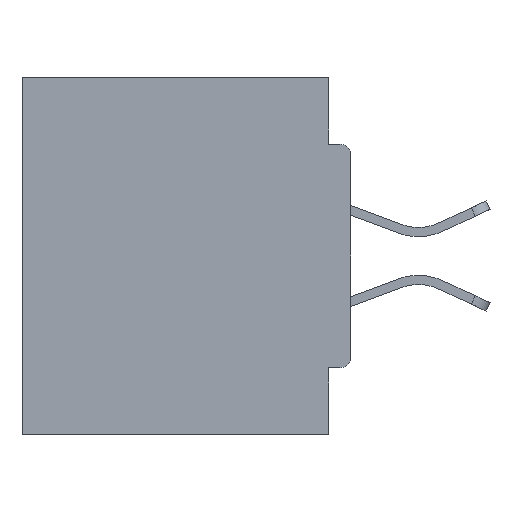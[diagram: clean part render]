
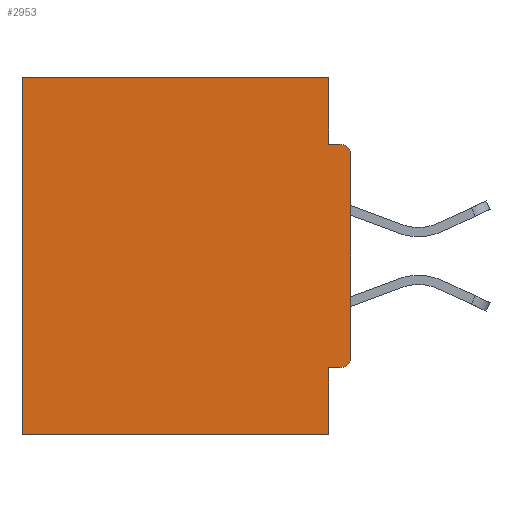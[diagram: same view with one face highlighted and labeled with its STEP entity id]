
A CAD part, left-side view. The second image highlights one B-rep face of the part: STEP entity #2953.
In plain terms, the highlighted planar face has unit normal (-1, 0, 0).
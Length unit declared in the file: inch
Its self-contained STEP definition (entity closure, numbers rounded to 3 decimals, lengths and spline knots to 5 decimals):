
#298 = AXIS2_PLACEMENT_3D ( 'NONE', #32883, #27693, #20295 ) ;
#1081 = CARTESIAN_POINT ( 'NONE',  ( 0.298, 0.015, -0.1085 ) ) ;
#1227 = EDGE_CURVE ( 'NONE', #9542, #20148, #21030, .T. ) ;
#1477 = VECTOR ( 'NONE', #25533, 39.37008 ) ;
#1722 = CARTESIAN_POINT ( 'NONE',  ( 0.298, 0.031, -0.5 ) ) ;
#2443 = EDGE_CURVE ( 'NONE', #21617, #32006, #15007, .T. ) ;
#2763 = PLANE ( 'NONE',  #298 ) ;
#2953 = ADVANCED_FACE ( 'NONE', ( #12989 ), #2763, .F. ) ;
#3527 = DIRECTION ( 'NONE',  ( -1., 0., 0. ) ) ;
#3782 = CARTESIAN_POINT ( 'NONE',  ( 0.298, 0.031, -0.4065 ) ) ;
#3964 = CARTESIAN_POINT ( 'NONE',  ( 0.298, 0.031, -0.0935 ) ) ;
#5133 = CARTESIAN_POINT ( 'NONE',  ( 0.298, 0.031, 0. ) ) ;
#5452 = VECTOR ( 'NONE', #10512, 39.37008 ) ;
#5731 = VERTEX_POINT ( 'NONE', #18969 ) ;
#5953 = AXIS2_PLACEMENT_3D ( 'NONE', #31043, #10849, #15747 ) ;
#6151 = CARTESIAN_POINT ( 'NONE',  ( 0.298, 0., -0.0935 ) ) ;
#6244 = ORIENTED_EDGE ( 'NONE', *, *, #21243, .T. ) ;
#6316 = CARTESIAN_POINT ( 'NONE',  ( 0.298, 0.031, -0.5 ) ) ;
#7752 = ORIENTED_EDGE ( 'NONE', *, *, #9714, .T. ) ;
#8006 = VERTEX_POINT ( 'NONE', #10909 ) ;
#8123 = LINE ( 'NONE', #1722, #21600 ) ;
#9542 = VERTEX_POINT ( 'NONE', #5133 ) ;
#9714 = EDGE_CURVE ( 'NONE', #16908, #8006, #12003, .T. ) ;
#9977 = CARTESIAN_POINT ( 'NONE',  ( 0.298, 0.46, -0.5 ) ) ;
#10256 = DIRECTION ( 'NONE',  ( 0., 1., 0. ) ) ;
#10280 = CARTESIAN_POINT ( 'NONE',  ( 0.298, 0.46, 0. ) ) ;
#10512 = DIRECTION ( 'NONE',  ( 0., 0., -1. ) ) ;
#10849 = DIRECTION ( 'NONE',  ( -1., 0., 0. ) ) ;
#10909 = CARTESIAN_POINT ( 'NONE',  ( 0.298, 0., -0.3915 ) ) ;
#10937 = DIRECTION ( 'NONE',  ( 0., -1., 0. ) ) ;
#11020 = ORIENTED_EDGE ( 'NONE', *, *, #1227, .F. ) ;
#11292 = VERTEX_POINT ( 'NONE', #3782 ) ;
#11693 = LINE ( 'NONE', #16660, #24375 ) ;
#12003 = CIRCLE ( 'NONE', #5953, 0.015 ) ;
#12701 = VECTOR ( 'NONE', #12727, 39.37008 ) ;
#12727 = DIRECTION ( 'NONE',  ( 0., 0., -1. ) ) ;
#12989 = FACE_OUTER_BOUND ( 'NONE', #31485, .T. ) ;
#13261 = CARTESIAN_POINT ( 'NONE',  ( 0.298, 0., -0.1085 ) ) ;
#13664 = ORIENTED_EDGE ( 'NONE', *, *, #16439, .F. ) ;
#14193 = VERTEX_POINT ( 'NONE', #13261 ) ;
#14961 = ORIENTED_EDGE ( 'NONE', *, *, #20725, .T. ) ;
#15007 = LINE ( 'NONE', #22960, #1477 ) ;
#15747 = DIRECTION ( 'NONE',  ( 0., 0., -1. ) ) ;
#16119 = LINE ( 'NONE', #30553, #24408 ) ;
#16439 = EDGE_CURVE ( 'NONE', #20148, #16506, #21629, .T. ) ;
#16506 = VERTEX_POINT ( 'NONE', #19716 ) ;
#16660 = CARTESIAN_POINT ( 'NONE',  ( 0.298, 0., 0. ) ) ;
#16773 = EDGE_CURVE ( 'NONE', #16908, #11292, #16119, .T. ) ;
#16908 = VERTEX_POINT ( 'NONE', #23781 ) ;
#18969 = CARTESIAN_POINT ( 'NONE',  ( 0.298, 0.46, 0. ) ) ;
#19121 = VECTOR ( 'NONE', #24846, 39.37008 ) ;
#19295 = DIRECTION ( 'NONE',  ( 0., 1., 0. ) ) ;
#19716 = CARTESIAN_POINT ( 'NONE',  ( 0.298, 0.015, -0.0935 ) ) ;
#20148 = VERTEX_POINT ( 'NONE', #3964 ) ;
#20295 = DIRECTION ( 'NONE',  ( 0., 0., -1. ) ) ;
#20707 = CARTESIAN_POINT ( 'NONE',  ( 0.298, 0.031, -0.5 ) ) ;
#20725 = EDGE_CURVE ( 'NONE', #9542, #5731, #11693, .T. ) ;
#21030 = LINE ( 'NONE', #20707, #12701 ) ;
#21243 = EDGE_CURVE ( 'NONE', #14193, #16506, #29960, .T. ) ;
#21294 = ORIENTED_EDGE ( 'NONE', *, *, #21366, .F. ) ;
#21360 = DIRECTION ( 'NONE',  ( 0., 0., -1. ) ) ;
#21366 = EDGE_CURVE ( 'NONE', #11292, #21617, #8123, .T. ) ;
#21478 = ORIENTED_EDGE ( 'NONE', *, *, #16773, .F. ) ;
#21600 = VECTOR ( 'NONE', #24675, 39.37008 ) ;
#21617 = VERTEX_POINT ( 'NONE', #6316 ) ;
#21629 = LINE ( 'NONE', #6151, #24028 ) ;
#22054 = LINE ( 'NONE', #10280, #5452 ) ;
#22960 = CARTESIAN_POINT ( 'NONE',  ( 0.298, 0., -0.5 ) ) ;
#23781 = CARTESIAN_POINT ( 'NONE',  ( 0.298, 0.015, -0.4065 ) ) ;
#24028 = VECTOR ( 'NONE', #10937, 39.37008 ) ;
#24254 = ORIENTED_EDGE ( 'NONE', *, *, #2443, .F. ) ;
#24375 = VECTOR ( 'NONE', #19295, 39.37008 ) ;
#24408 = VECTOR ( 'NONE', #10256, 39.37008 ) ;
#24675 = DIRECTION ( 'NONE',  ( 0., 0., -1. ) ) ;
#24846 = DIRECTION ( 'NONE',  ( 0., 0., -1. ) ) ;
#24960 = EDGE_CURVE ( 'NONE', #14193, #8006, #32675, .T. ) ;
#25461 = ORIENTED_EDGE ( 'NONE', *, *, #28849, .T. ) ;
#25533 = DIRECTION ( 'NONE',  ( 0., 1., 0. ) ) ;
#27337 = AXIS2_PLACEMENT_3D ( 'NONE', #1081, #3527, #21360 ) ;
#27693 = DIRECTION ( 'NONE',  ( 1., 0., 0. ) ) ;
#28849 = EDGE_CURVE ( 'NONE', #5731, #32006, #22054, .T. ) ;
#29960 = CIRCLE ( 'NONE', #27337, 0.015 ) ;
#30066 = CARTESIAN_POINT ( 'NONE',  ( 0.298, 0., 0. ) ) ;
#30553 = CARTESIAN_POINT ( 'NONE',  ( 0.298, 0., -0.4065 ) ) ;
#31043 = CARTESIAN_POINT ( 'NONE',  ( 0.298, 0.015, -0.3915 ) ) ;
#31485 = EDGE_LOOP ( 'NONE', ( #6244, #13664, #11020, #14961, #25461, #24254, #21294, #21478, #7752, #32307 ) ) ;
#32006 = VERTEX_POINT ( 'NONE', #9977 ) ;
#32307 = ORIENTED_EDGE ( 'NONE', *, *, #24960, .F. ) ;
#32675 = LINE ( 'NONE', #30066, #19121 ) ;
#32883 = CARTESIAN_POINT ( 'NONE',  ( 0.298, 0., 0. ) ) ;
